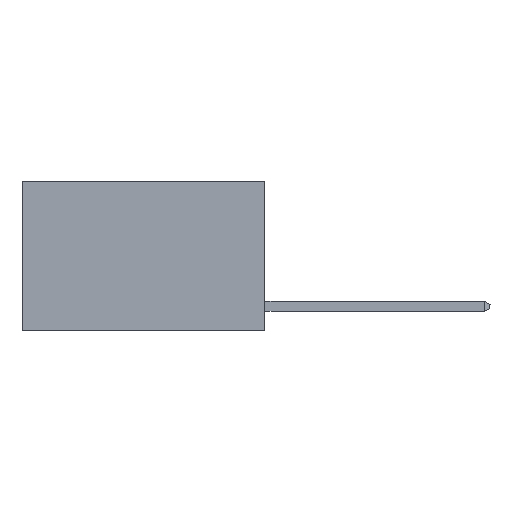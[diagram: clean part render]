
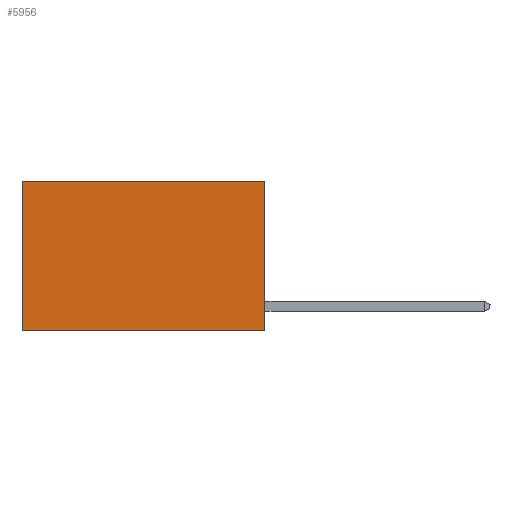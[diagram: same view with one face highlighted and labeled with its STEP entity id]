
A CAD part, left-side view. The second image highlights one B-rep face of the part: STEP entity #5956.
In plain terms, the highlighted planar face has unit normal (-1, 0, 0).
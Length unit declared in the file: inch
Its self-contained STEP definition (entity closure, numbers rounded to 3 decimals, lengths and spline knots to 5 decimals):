
#452 = CARTESIAN_POINT ( 'NONE',  ( 0.2625, 0., -0.37 ) ) ;
#680 = ORIENTED_EDGE ( 'NONE', *, *, #10039, .F. ) ;
#781 = EDGE_LOOP ( 'NONE', ( #2352, #10041, #680, #9393 ) ) ;
#2022 = EDGE_CURVE ( 'NONE', #9927, #8389, #3252, .T. ) ;
#2352 = ORIENTED_EDGE ( 'NONE', *, *, #9604, .T. ) ;
#2461 = AXIS2_PLACEMENT_3D ( 'NONE', #2858, #7108, #8917 ) ;
#2587 = VECTOR ( 'NONE', #9120, 39.37008 ) ;
#2827 = PLANE ( 'NONE',  #2461 ) ;
#2858 = CARTESIAN_POINT ( 'NONE',  ( 0.2625, 0., 0. ) ) ;
#3252 = LINE ( 'NONE', #452, #2587 ) ;
#3846 = VERTEX_POINT ( 'NONE', #5566 ) ;
#4323 = CARTESIAN_POINT ( 'NONE',  ( 0.2625, 0., -0.37 ) ) ;
#4429 = VECTOR ( 'NONE', #9473, 39.37008 ) ;
#4631 = LINE ( 'NONE', #9708, #8010 ) ;
#5172 = CARTESIAN_POINT ( 'NONE',  ( 0.2625, 0., 0. ) ) ;
#5566 = CARTESIAN_POINT ( 'NONE',  ( 0.2625, 0.6, 0. ) ) ;
#5956 = ADVANCED_FACE ( 'NONE', ( #8372 ), #2827, .F. ) ;
#5977 = VECTOR ( 'NONE', #8927, 39.37008 ) ;
#7108 = DIRECTION ( 'NONE',  ( 1., 0., 0. ) ) ;
#7287 = LINE ( 'NONE', #5172, #4429 ) ;
#7975 = EDGE_CURVE ( 'NONE', #9586, #3846, #7287, .T. ) ;
#8010 = VECTOR ( 'NONE', #8706, 39.37008 ) ;
#8329 = CARTESIAN_POINT ( 'NONE',  ( 0.2625, 0.6, -0.37 ) ) ;
#8372 = FACE_OUTER_BOUND ( 'NONE', #781, .T. ) ;
#8389 = VERTEX_POINT ( 'NONE', #8329 ) ;
#8531 = LINE ( 'NONE', #8850, #5977 ) ;
#8706 = DIRECTION ( 'NONE',  ( 0., 0., -1. ) ) ;
#8850 = CARTESIAN_POINT ( 'NONE',  ( 0.2625, 0., 0. ) ) ;
#8917 = DIRECTION ( 'NONE',  ( 0., 0., -1. ) ) ;
#8927 = DIRECTION ( 'NONE',  ( 0., 0., -1. ) ) ;
#9120 = DIRECTION ( 'NONE',  ( 0., 1., 0. ) ) ;
#9393 = ORIENTED_EDGE ( 'NONE', *, *, #7975, .T. ) ;
#9473 = DIRECTION ( 'NONE',  ( 0., 1., 0. ) ) ;
#9586 = VERTEX_POINT ( 'NONE', #10392 ) ;
#9604 = EDGE_CURVE ( 'NONE', #3846, #8389, #4631, .T. ) ;
#9708 = CARTESIAN_POINT ( 'NONE',  ( 0.2625, 0.6, 0. ) ) ;
#9927 = VERTEX_POINT ( 'NONE', #4323 ) ;
#10039 = EDGE_CURVE ( 'NONE', #9586, #9927, #8531, .T. ) ;
#10041 = ORIENTED_EDGE ( 'NONE', *, *, #2022, .F. ) ;
#10392 = CARTESIAN_POINT ( 'NONE',  ( 0.2625, 0., 0. ) ) ;
